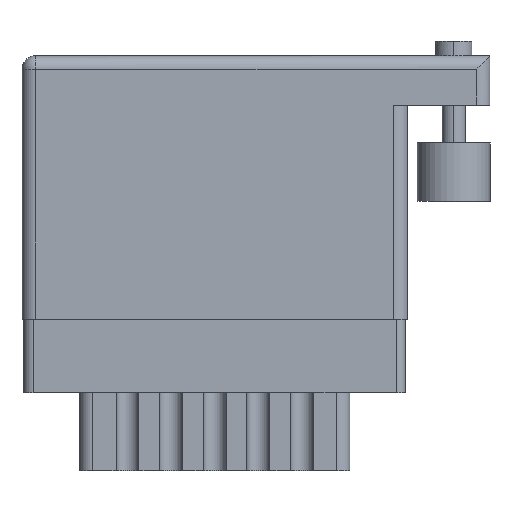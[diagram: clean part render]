
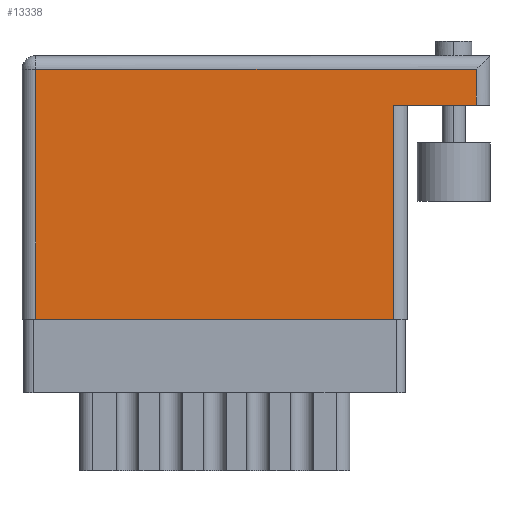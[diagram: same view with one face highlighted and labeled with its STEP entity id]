
A CAD part, front view. The second image highlights one B-rep face of the part: STEP entity #13338.
In plain terms, the highlighted face is planar.
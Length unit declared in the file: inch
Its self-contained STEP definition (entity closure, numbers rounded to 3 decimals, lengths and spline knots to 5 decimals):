
#172 = LINE ( 'NONE', #13412, #11900 ) ;
#503 = CARTESIAN_POINT ( 'NONE',  ( 1.562, 0.736, 0. ) ) ;
#848 = VECTOR ( 'NONE', #19260, 39.37008 ) ;
#945 = ORIENTED_EDGE ( 'NONE', *, *, #12572, .T. ) ;
#946 = CARTESIAN_POINT ( 'NONE',  ( 1.278, 0., 0. ) ) ;
#2092 = CARTESIAN_POINT ( 'NONE',  ( 0.047, 0.859, 0. ) ) ;
#2231 = DIRECTION ( 'NONE',  ( 1., 0., 0. ) ) ;
#2721 = VERTEX_POINT ( 'NONE', #15014 ) ;
#2899 = CARTESIAN_POINT ( 'NONE',  ( 0.047, 0., 0. ) ) ;
#3002 = CARTESIAN_POINT ( 'NONE',  ( 1.562, 0.906, 0. ) ) ;
#3375 = EDGE_LOOP ( 'NONE', ( #9508, #12415, #11006, #9272, #7172, #945 ) ) ;
#3522 = CARTESIAN_POINT ( 'NONE',  ( 0., 0., 0. ) ) ;
#4467 = DIRECTION ( 'NONE',  ( 0., 1., 0. ) ) ;
#5333 = VECTOR ( 'NONE', #4467, 39.37008 ) ;
#5384 = LINE ( 'NONE', #13764, #10137 ) ;
#7172 = ORIENTED_EDGE ( 'NONE', *, *, #16002, .T. ) ;
#7188 = EDGE_CURVE ( 'NONE', #20037, #9062, #5384, .T. ) ;
#7391 = DIRECTION ( 'NONE',  ( -1., 0., 0. ) ) ;
#7436 = DIRECTION ( 'NONE',  ( 0., -1., 0. ) ) ;
#7764 = VERTEX_POINT ( 'NONE', #946 ) ;
#8026 = DIRECTION ( 'NONE',  ( -1., 0., 0. ) ) ;
#9062 = VERTEX_POINT ( 'NONE', #10844 ) ;
#9216 = LINE ( 'NONE', #19220, #5333 ) ;
#9272 = ORIENTED_EDGE ( 'NONE', *, *, #18084, .T. ) ;
#9288 = VERTEX_POINT ( 'NONE', #2092 ) ;
#9477 = LINE ( 'NONE', #3002, #848 ) ;
#9508 = ORIENTED_EDGE ( 'NONE', *, *, #10372, .T. ) ;
#10137 = VECTOR ( 'NONE', #18732, 39.37008 ) ;
#10372 = EDGE_CURVE ( 'NONE', #2721, #7764, #18491, .T. ) ;
#10620 = VERTEX_POINT ( 'NONE', #18020 ) ;
#10711 = FACE_OUTER_BOUND ( 'NONE', #3375, .T. ) ;
#10844 = CARTESIAN_POINT ( 'NONE',  ( 1.278, 0.736, 0. ) ) ;
#11006 = ORIENTED_EDGE ( 'NONE', *, *, #7188, .F. ) ;
#11900 = VECTOR ( 'NONE', #8026, 39.37008 ) ;
#12415 = ORIENTED_EDGE ( 'NONE', *, *, #18915, .T. ) ;
#12572 = EDGE_CURVE ( 'NONE', #9288, #2721, #17649, .T. ) ;
#13338 = ADVANCED_FACE ( 'NONE', ( #10711 ), #15561, .F. ) ;
#13412 = CARTESIAN_POINT ( 'NONE',  ( 0., 0.859, 0. ) ) ;
#13764 = CARTESIAN_POINT ( 'NONE',  ( 1.609, 0.736, 0. ) ) ;
#14698 = VECTOR ( 'NONE', #2231, 39.37008 ) ;
#15014 = CARTESIAN_POINT ( 'NONE',  ( 0.047, 0., 0. ) ) ;
#15561 = PLANE ( 'NONE',  #18347 ) ;
#16002 = EDGE_CURVE ( 'NONE', #10620, #9288, #172, .T. ) ;
#17286 = DIRECTION ( 'NONE',  ( 0., 0., -1. ) ) ;
#17649 = LINE ( 'NONE', #2899, #20796 ) ;
#18020 = CARTESIAN_POINT ( 'NONE',  ( 1.562, 0.859, 0. ) ) ;
#18084 = EDGE_CURVE ( 'NONE', #20037, #10620, #9477, .T. ) ;
#18347 = AXIS2_PLACEMENT_3D ( 'NONE', #20733, #17286, #7391 ) ;
#18491 = LINE ( 'NONE', #3522, #14698 ) ;
#18732 = DIRECTION ( 'NONE',  ( -1., 0., 0. ) ) ;
#18915 = EDGE_CURVE ( 'NONE', #7764, #9062, #9216, .T. ) ;
#19220 = CARTESIAN_POINT ( 'NONE',  ( 1.278, 0.736, 0. ) ) ;
#19260 = DIRECTION ( 'NONE',  ( 0., 1., 0. ) ) ;
#20037 = VERTEX_POINT ( 'NONE', #503 ) ;
#20733 = CARTESIAN_POINT ( 'NONE',  ( 0., 0.906, 0. ) ) ;
#20796 = VECTOR ( 'NONE', #7436, 39.37008 ) ;
